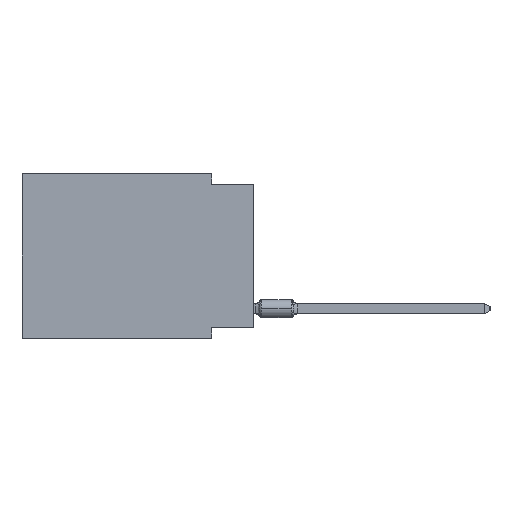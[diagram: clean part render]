
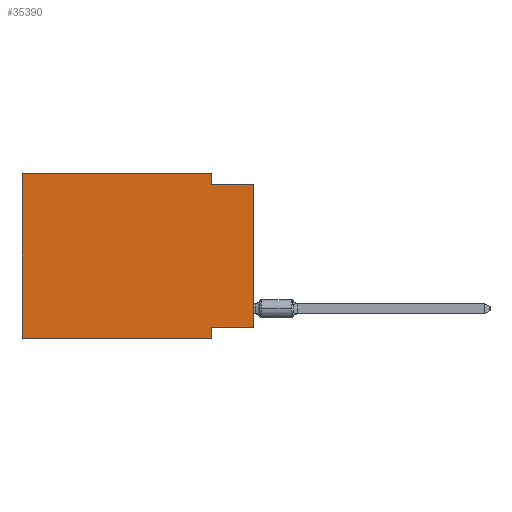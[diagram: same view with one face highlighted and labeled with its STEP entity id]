
A CAD part, left-side view. The second image highlights one B-rep face of the part: STEP entity #35390.
In plain terms, the highlighted planar face has unit normal (-1, 0, 0).
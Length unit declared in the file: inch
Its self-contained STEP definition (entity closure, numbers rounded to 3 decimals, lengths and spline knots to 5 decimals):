
#565 = ORIENTED_EDGE ( 'NONE', *, *, #24412, .F. ) ;
#1295 = CARTESIAN_POINT ( 'NONE',  ( 0., 0.55, 0. ) ) ;
#1444 = ORIENTED_EDGE ( 'NONE', *, *, #31636, .F. ) ;
#2474 = DIRECTION ( 'NONE',  ( 0., 0., -1. ) ) ;
#2636 = EDGE_CURVE ( 'NONE', #8759, #45831, #44032, .T. ) ;
#3009 = LINE ( 'NONE', #49594, #15399 ) ;
#3092 = VERTEX_POINT ( 'NONE', #15395 ) ;
#3308 = DIRECTION ( 'NONE',  ( 0., 0., 1. ) ) ;
#3863 = VECTOR ( 'NONE', #25214, 39.37008 ) ;
#7557 = VECTOR ( 'NONE', #36812, 39.37008 ) ;
#7819 = EDGE_CURVE ( 'NONE', #9016, #3092, #3009, .T. ) ;
#8759 = VERTEX_POINT ( 'NONE', #12941 ) ;
#8818 = DIRECTION ( 'NONE',  ( 0., -1., 0. ) ) ;
#9016 = VERTEX_POINT ( 'NONE', #22992 ) ;
#9056 = DIRECTION ( 'NONE',  ( 0., -1., 0. ) ) ;
#9524 = ORIENTED_EDGE ( 'NONE', *, *, #38415, .F. ) ;
#9528 = CARTESIAN_POINT ( 'NONE',  ( 0., 0.55, -0.39 ) ) ;
#9571 = VERTEX_POINT ( 'NONE', #31654 ) ;
#10335 = ORIENTED_EDGE ( 'NONE', *, *, #37208, .F. ) ;
#12941 = CARTESIAN_POINT ( 'NONE',  ( 0., 0.55, -0.39 ) ) ;
#13187 = ORIENTED_EDGE ( 'NONE', *, *, #46679, .T. ) ;
#13875 = CARTESIAN_POINT ( 'NONE',  ( 0., 0., -0.365 ) ) ;
#14524 = ORIENTED_EDGE ( 'NONE', *, *, #16658, .F. ) ;
#15395 = CARTESIAN_POINT ( 'NONE',  ( 0., 0.1, -0.025 ) ) ;
#15399 = VECTOR ( 'NONE', #29666, 39.37008 ) ;
#16351 = LINE ( 'NONE', #1295, #17578 ) ;
#16658 = EDGE_CURVE ( 'NONE', #30095, #45831, #17795, .T. ) ;
#16776 = VECTOR ( 'NONE', #40241, 39.37008 ) ;
#17188 = EDGE_LOOP ( 'NONE', ( #13187, #565, #42844, #10335, #1444, #27171, #14524, #9524 ) ) ;
#17578 = VECTOR ( 'NONE', #9056, 39.37008 ) ;
#17795 = LINE ( 'NONE', #25373, #29837 ) ;
#18268 = AXIS2_PLACEMENT_3D ( 'NONE', #41128, #33572, #44924 ) ;
#18711 = PLANE ( 'NONE',  #18268 ) ;
#20301 = VECTOR ( 'NONE', #8818, 39.37008 ) ;
#20414 = LINE ( 'NONE', #46877, #20301 ) ;
#21875 = CARTESIAN_POINT ( 'NONE',  ( 0., 0., -0.025 ) ) ;
#22660 = CARTESIAN_POINT ( 'NONE',  ( 0., 0.55, 0. ) ) ;
#22992 = CARTESIAN_POINT ( 'NONE',  ( 0., 0.1, 0. ) ) ;
#23136 = CARTESIAN_POINT ( 'NONE',  ( 0., 0.55, 0. ) ) ;
#24412 = EDGE_CURVE ( 'NONE', #3092, #37403, #20414, .T. ) ;
#24609 = CARTESIAN_POINT ( 'NONE',  ( 0., 0.1, -0.365 ) ) ;
#24961 = CARTESIAN_POINT ( 'NONE',  ( 0., 0., 0. ) ) ;
#25214 = DIRECTION ( 'NONE',  ( 0., 1., 0. ) ) ;
#25373 = CARTESIAN_POINT ( 'NONE',  ( 0., 0.1, -0.39 ) ) ;
#25962 = LINE ( 'NONE', #13875, #3863 ) ;
#27171 = ORIENTED_EDGE ( 'NONE', *, *, #2636, .T. ) ;
#29666 = DIRECTION ( 'NONE',  ( 0., 0., -1. ) ) ;
#29837 = VECTOR ( 'NONE', #2474, 39.37008 ) ;
#30095 = VERTEX_POINT ( 'NONE', #24609 ) ;
#31636 = EDGE_CURVE ( 'NONE', #8759, #49651, #34492, .T. ) ;
#31654 = CARTESIAN_POINT ( 'NONE',  ( 0., 0., -0.365 ) ) ;
#33523 = LINE ( 'NONE', #24961, #7557 ) ;
#33572 = DIRECTION ( 'NONE',  ( 1., 0., 0. ) ) ;
#34492 = LINE ( 'NONE', #22660, #40775 ) ;
#35390 = ADVANCED_FACE ( 'NONE', ( #44682 ), #18711, .F. ) ;
#36812 = DIRECTION ( 'NONE',  ( 0., 0., 1. ) ) ;
#37208 = EDGE_CURVE ( 'NONE', #49651, #9016, #16351, .T. ) ;
#37403 = VERTEX_POINT ( 'NONE', #21875 ) ;
#38415 = EDGE_CURVE ( 'NONE', #9571, #30095, #25962, .T. ) ;
#40241 = DIRECTION ( 'NONE',  ( 0., -1., 0. ) ) ;
#40775 = VECTOR ( 'NONE', #3308, 39.37008 ) ;
#41128 = CARTESIAN_POINT ( 'NONE',  ( 0., 0.55, 0. ) ) ;
#42844 = ORIENTED_EDGE ( 'NONE', *, *, #7819, .F. ) ;
#44032 = LINE ( 'NONE', #9528, #16776 ) ;
#44682 = FACE_OUTER_BOUND ( 'NONE', #17188, .T. ) ;
#44924 = DIRECTION ( 'NONE',  ( 0., 0., -1. ) ) ;
#45831 = VERTEX_POINT ( 'NONE', #46035 ) ;
#46035 = CARTESIAN_POINT ( 'NONE',  ( 0., 0.1, -0.39 ) ) ;
#46679 = EDGE_CURVE ( 'NONE', #9571, #37403, #33523, .T. ) ;
#46877 = CARTESIAN_POINT ( 'NONE',  ( 0., 0., -0.025 ) ) ;
#49594 = CARTESIAN_POINT ( 'NONE',  ( 0., 0.1, 0. ) ) ;
#49651 = VERTEX_POINT ( 'NONE', #23136 ) ;
